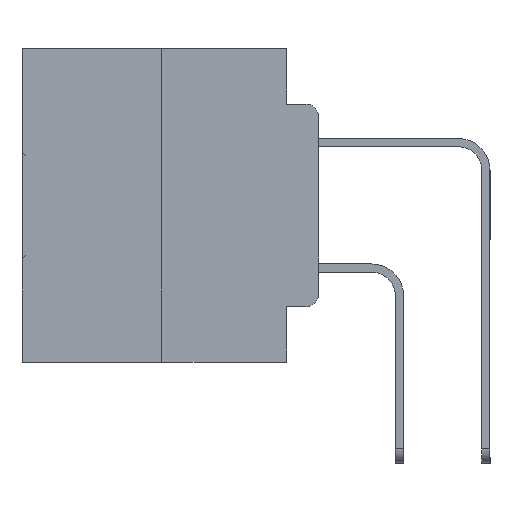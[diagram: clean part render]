
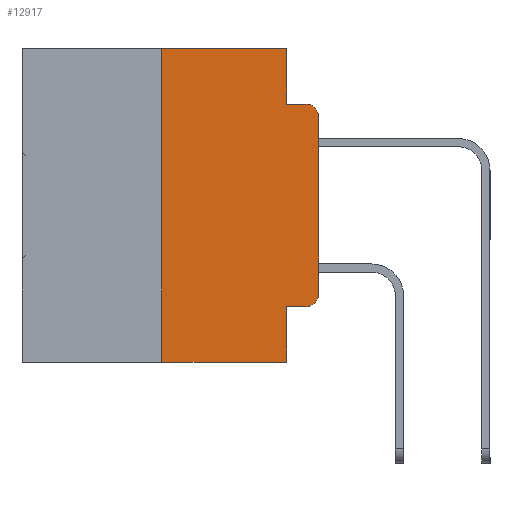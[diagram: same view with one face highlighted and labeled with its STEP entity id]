
A CAD part, left-side view. The second image highlights one B-rep face of the part: STEP entity #12917.
In plain terms, the highlighted planar face has unit normal (-1, 0, 0).
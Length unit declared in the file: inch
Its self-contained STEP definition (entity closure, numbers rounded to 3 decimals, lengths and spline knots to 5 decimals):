
#17 = CARTESIAN_POINT ( 'NONE',  ( 0., 0.25, -0.5 ) ) ;
#273 = CARTESIAN_POINT ( 'NONE',  ( 0., 0.473, 0. ) ) ;
#300 = VERTEX_POINT ( 'NONE', #10084 ) ;
#865 = ORIENTED_EDGE ( 'NONE', *, *, #20247, .T. ) ;
#2541 = CARTESIAN_POINT ( 'NONE',  ( 0., 0.473, 0. ) ) ;
#2996 = CARTESIAN_POINT ( 'NONE',  ( 0., 0., -0.3915 ) ) ;
#3166 = DIRECTION ( 'NONE',  ( 0., -1., 0. ) ) ;
#3371 = VERTEX_POINT ( 'NONE', #11243 ) ;
#3620 = CARTESIAN_POINT ( 'NONE',  ( 0., 0.473, -0.5 ) ) ;
#4275 = ORIENTED_EDGE ( 'NONE', *, *, #31960, .T. ) ;
#4665 = CARTESIAN_POINT ( 'NONE',  ( 0., 0., 0. ) ) ;
#4956 = ORIENTED_EDGE ( 'NONE', *, *, #5572, .F. ) ;
#5572 = EDGE_CURVE ( 'NONE', #300, #22469, #19594, .T. ) ;
#5747 = CARTESIAN_POINT ( 'NONE',  ( 0., 0.051, -0.0885 ) ) ;
#6087 = LINE ( 'NONE', #19464, #12822 ) ;
#6803 = EDGE_CURVE ( 'NONE', #3371, #28757, #27696, .T. ) ;
#6952 = ORIENTED_EDGE ( 'NONE', *, *, #18596, .F. ) ;
#8169 = VERTEX_POINT ( 'NONE', #2996 ) ;
#8521 = EDGE_CURVE ( 'NONE', #19114, #300, #23278, .T. ) ;
#8525 = VECTOR ( 'NONE', #12646, 39.37008 ) ;
#8607 = DIRECTION ( 'NONE',  ( -1., 0., 0. ) ) ;
#9292 = VECTOR ( 'NONE', #16262, 39.37008 ) ;
#9366 = VERTEX_POINT ( 'NONE', #13934 ) ;
#10072 = LINE ( 'NONE', #3620, #9292 ) ;
#10084 = CARTESIAN_POINT ( 'NONE',  ( 0., 0.25, 0. ) ) ;
#10571 = CARTESIAN_POINT ( 'NONE',  ( 0., 0.25, 0. ) ) ;
#11243 = CARTESIAN_POINT ( 'NONE',  ( 0., 0.051, -0.4115 ) ) ;
#12335 = DIRECTION ( 'NONE',  ( 0., 0., 1. ) ) ;
#12590 = CARTESIAN_POINT ( 'NONE',  ( 0., 0.02, -0.3915 ) ) ;
#12640 = CARTESIAN_POINT ( 'NONE',  ( 0., 0.051, 0. ) ) ;
#12646 = DIRECTION ( 'NONE',  ( 0., 0., -1. ) ) ;
#12784 = DIRECTION ( 'NONE',  ( 0., 0., -1. ) ) ;
#12822 = VECTOR ( 'NONE', #21977, 39.37008 ) ;
#12886 = ORIENTED_EDGE ( 'NONE', *, *, #16140, .T. ) ;
#12917 = ADVANCED_FACE ( 'NONE', ( #20879 ), #20198, .F. ) ;
#13891 = VECTOR ( 'NONE', #3166, 39.37008 ) ;
#13934 = CARTESIAN_POINT ( 'NONE',  ( 0., 0.02, -0.4115 ) ) ;
#14879 = ORIENTED_EDGE ( 'NONE', *, *, #29267, .T. ) ;
#14982 = ORIENTED_EDGE ( 'NONE', *, *, #30925, .T. ) ;
#15114 = DIRECTION ( 'NONE',  ( 0., 0., -1. ) ) ;
#15646 = ORIENTED_EDGE ( 'NONE', *, *, #16936, .F. ) ;
#16140 = EDGE_CURVE ( 'NONE', #19114, #28757, #10072, .T. ) ;
#16262 = DIRECTION ( 'NONE',  ( 0., -1., 0. ) ) ;
#16648 = ORIENTED_EDGE ( 'NONE', *, *, #6803, .F. ) ;
#16936 = EDGE_CURVE ( 'NONE', #22469, #31587, #6087, .T. ) ;
#17316 = AXIS2_PLACEMENT_3D ( 'NONE', #12590, #30050, #15114 ) ;
#17646 = LINE ( 'NONE', #4665, #23516 ) ;
#18596 = EDGE_CURVE ( 'NONE', #31587, #22429, #27936, .T. ) ;
#18958 = DIRECTION ( 'NONE',  ( 0., -1., 0. ) ) ;
#19114 = VERTEX_POINT ( 'NONE', #17 ) ;
#19464 = CARTESIAN_POINT ( 'NONE',  ( 0., 0.051, 0. ) ) ;
#19594 = LINE ( 'NONE', #273, #26241 ) ;
#20198 = PLANE ( 'NONE',  #29323 ) ;
#20247 = EDGE_CURVE ( 'NONE', #22593, #22429, #31382, .T. ) ;
#20879 = FACE_OUTER_BOUND ( 'NONE', #30332, .T. ) ;
#21977 = DIRECTION ( 'NONE',  ( 0., 0., -1. ) ) ;
#22414 = VECTOR ( 'NONE', #18958, 39.37008 ) ;
#22429 = VERTEX_POINT ( 'NONE', #27389 ) ;
#22469 = VERTEX_POINT ( 'NONE', #12640 ) ;
#22593 = VERTEX_POINT ( 'NONE', #23115 ) ;
#23115 = CARTESIAN_POINT ( 'NONE',  ( 0., 0., -0.1085 ) ) ;
#23278 = LINE ( 'NONE', #10571, #29910 ) ;
#23516 = VECTOR ( 'NONE', #12335, 39.37008 ) ;
#23590 = CARTESIAN_POINT ( 'NONE',  ( 0., 0.02, -0.1085 ) ) ;
#24051 = CARTESIAN_POINT ( 'NONE',  ( 0., 0.051, -0.0885 ) ) ;
#25508 = DIRECTION ( 'NONE',  ( 0., -1., 0. ) ) ;
#26110 = DIRECTION ( 'NONE',  ( 0., 0., -1. ) ) ;
#26241 = VECTOR ( 'NONE', #25508, 39.37008 ) ;
#26385 = ORIENTED_EDGE ( 'NONE', *, *, #8521, .F. ) ;
#27389 = CARTESIAN_POINT ( 'NONE',  ( 0., 0.02, -0.0885 ) ) ;
#27612 = CARTESIAN_POINT ( 'NONE',  ( 0., 0.051, 0. ) ) ;
#27613 = CIRCLE ( 'NONE', #17316, 0.02 ) ;
#27696 = LINE ( 'NONE', #27612, #8525 ) ;
#27749 = DIRECTION ( 'NONE',  ( 1., 0., 0. ) ) ;
#27936 = LINE ( 'NONE', #5747, #13891 ) ;
#28164 = DIRECTION ( 'NONE',  ( 0., 0., 1. ) ) ;
#28276 = LINE ( 'NONE', #28986, #22414 ) ;
#28757 = VERTEX_POINT ( 'NONE', #32467 ) ;
#28986 = CARTESIAN_POINT ( 'NONE',  ( 0., 0.051, -0.4115 ) ) ;
#29267 = EDGE_CURVE ( 'NONE', #9366, #8169, #27613, .T. ) ;
#29323 = AXIS2_PLACEMENT_3D ( 'NONE', #2541, #27749, #12784 ) ;
#29910 = VECTOR ( 'NONE', #28164, 39.37008 ) ;
#30050 = DIRECTION ( 'NONE',  ( -1., 0., 0. ) ) ;
#30332 = EDGE_LOOP ( 'NONE', ( #4275, #865, #6952, #15646, #4956, #26385, #12886, #16648, #14982, #14879 ) ) ;
#30925 = EDGE_CURVE ( 'NONE', #3371, #9366, #28276, .T. ) ;
#31113 = AXIS2_PLACEMENT_3D ( 'NONE', #23590, #8607, #26110 ) ;
#31382 = CIRCLE ( 'NONE', #31113, 0.02 ) ;
#31587 = VERTEX_POINT ( 'NONE', #24051 ) ;
#31960 = EDGE_CURVE ( 'NONE', #8169, #22593, #17646, .T. ) ;
#32467 = CARTESIAN_POINT ( 'NONE',  ( 0., 0.051, -0.5 ) ) ;
